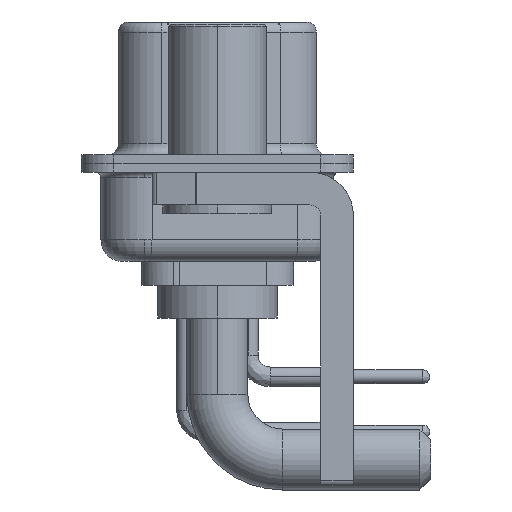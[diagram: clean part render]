
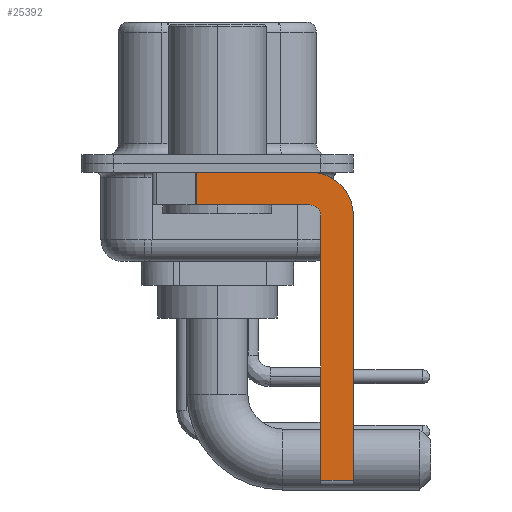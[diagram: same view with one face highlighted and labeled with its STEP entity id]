
A CAD part, left-side view. The second image highlights one B-rep face of the part: STEP entity #25392.
In plain terms, the highlighted planar face has unit normal (-1, 0, 0).
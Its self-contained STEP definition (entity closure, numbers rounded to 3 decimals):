
#277 = AXIS2_PLACEMENT_3D ( 'NONE', #25012, #14095, #2084 ) ;
#881 = VERTEX_POINT ( 'NONE', #25821 ) ;
#1530 = DIRECTION ( 'NONE',  ( 0., 0., -1. ) ) ;
#1732 = CARTESIAN_POINT ( 'NONE',  ( -2.9, -6.25, -2.4 ) ) ;
#1864 = DIRECTION ( 'NONE',  ( 0., -1., 0. ) ) ;
#2084 = DIRECTION ( 'NONE',  ( 0., 0., 1. ) ) ;
#2325 = VERTEX_POINT ( 'NONE', #13646 ) ;
#2996 = VECTOR ( 'NONE', #1864, 1000. ) ;
#3600 = ORIENTED_EDGE ( 'NONE', *, *, #15627, .F. ) ;
#5427 = DIRECTION ( 'NONE',  ( 0., 0., -1. ) ) ;
#5645 = VECTOR ( 'NONE', #12562, 1000. ) ;
#6056 = CARTESIAN_POINT ( 'NONE',  ( -2.9, -6.25, -14.55 ) ) ;
#6804 = CIRCLE ( 'NONE', #277, 0.5 ) ;
#6904 = EDGE_CURVE ( 'NONE', #26498, #11648, #24793, .T. ) ;
#7763 = ORIENTED_EDGE ( 'NONE', *, *, #18402, .F. ) ;
#7865 = CARTESIAN_POINT ( 'NONE',  ( -2.9, 3., -0.4 ) ) ;
#7997 = LINE ( 'NONE', #7865, #25179 ) ;
#8092 = VERTEX_POINT ( 'NONE', #1732 ) ;
#8400 = EDGE_LOOP ( 'NONE', ( #18350, #20462, #3600, #20736, #19593, #17802, #7763, #24963 ) ) ;
#9025 = CIRCLE ( 'NONE', #20380, 2. ) ;
#9372 = DIRECTION ( 'NONE',  ( 1., 0., 0. ) ) ;
#9666 = VERTEX_POINT ( 'NONE', #16493 ) ;
#10120 = CARTESIAN_POINT ( 'NONE',  ( -2.9, -4.25, -1.9 ) ) ;
#10349 = CARTESIAN_POINT ( 'NONE',  ( -2.9, 0.978, -1.9 ) ) ;
#11109 = DIRECTION ( 'NONE',  ( 0., 0., -1. ) ) ;
#11648 = VERTEX_POINT ( 'NONE', #6056 ) ;
#12027 = AXIS2_PLACEMENT_3D ( 'NONE', #26313, #9372, #5427 ) ;
#12562 = DIRECTION ( 'NONE',  ( 0., 1., 0. ) ) ;
#12820 = CARTESIAN_POINT ( 'NONE',  ( -2.9, -4.25, -2.4 ) ) ;
#13646 = CARTESIAN_POINT ( 'NONE',  ( -2.9, -4.25, -0.4 ) ) ;
#13947 = LINE ( 'NONE', #22413, #15837 ) ;
#14095 = DIRECTION ( 'NONE',  ( -1., 0., 0. ) ) ;
#14856 = CARTESIAN_POINT ( 'NONE',  ( -2.9, -4.75, -14.55 ) ) ;
#15075 = DIRECTION ( 'NONE',  ( 0., 0., 1. ) ) ;
#15415 = EDGE_CURVE ( 'NONE', #26498, #881, #25723, .T. ) ;
#15627 = EDGE_CURVE ( 'NONE', #25010, #16134, #26785, .T. ) ;
#15837 = VECTOR ( 'NONE', #1530, 1000. ) ;
#16134 = VERTEX_POINT ( 'NONE', #10349 ) ;
#16237 = VECTOR ( 'NONE', #11109, 1000. ) ;
#16348 = DIRECTION ( 'NONE',  ( 0., -1., 0. ) ) ;
#16493 = CARTESIAN_POINT ( 'NONE',  ( -2.9, 0.978, -0.4 ) ) ;
#17627 = CARTESIAN_POINT ( 'NONE',  ( -2.9, -4.25, -1.9 ) ) ;
#17802 = ORIENTED_EDGE ( 'NONE', *, *, #6904, .T. ) ;
#18350 = ORIENTED_EDGE ( 'NONE', *, *, #26889, .F. ) ;
#18402 = EDGE_CURVE ( 'NONE', #8092, #11648, #21763, .T. ) ;
#19593 = ORIENTED_EDGE ( 'NONE', *, *, #15415, .F. ) ;
#19669 = DIRECTION ( 'NONE',  ( 0., 0., -1. ) ) ;
#20380 = AXIS2_PLACEMENT_3D ( 'NONE', #12820, #23762, #19669 ) ;
#20462 = ORIENTED_EDGE ( 'NONE', *, *, #20621, .T. ) ;
#20585 = CARTESIAN_POINT ( 'NONE',  ( -2.9, -4.25, -14.55 ) ) ;
#20621 = EDGE_CURVE ( 'NONE', #9666, #16134, #13947, .T. ) ;
#20736 = ORIENTED_EDGE ( 'NONE', *, *, #23852, .F. ) ;
#21504 = CARTESIAN_POINT ( 'NONE',  ( -2.9, -6.25, -2.4 ) ) ;
#21633 = CARTESIAN_POINT ( 'NONE',  ( -2.9, -4.75, -14.8 ) ) ;
#21686 = PLANE ( 'NONE',  #12027 ) ;
#21763 = LINE ( 'NONE', #21504, #16237 ) ;
#22413 = CARTESIAN_POINT ( 'NONE',  ( -2.9, 0.978, -1.9 ) ) ;
#22642 = VECTOR ( 'NONE', #15075, 1000. ) ;
#23762 = DIRECTION ( 'NONE',  ( 1., 0., 0. ) ) ;
#23852 = EDGE_CURVE ( 'NONE', #881, #25010, #6804, .T. ) ;
#24793 = LINE ( 'NONE', #20585, #2996 ) ;
#24963 = ORIENTED_EDGE ( 'NONE', *, *, #26171, .F. ) ;
#25010 = VERTEX_POINT ( 'NONE', #17627 ) ;
#25012 = CARTESIAN_POINT ( 'NONE',  ( -2.9, -4.25, -2.4 ) ) ;
#25179 = VECTOR ( 'NONE', #16348, 1000. ) ;
#25392 = ADVANCED_FACE ( 'NONE', ( #26177 ), #21686, .F. ) ;
#25723 = LINE ( 'NONE', #21633, #22642 ) ;
#25821 = CARTESIAN_POINT ( 'NONE',  ( -2.9, -4.75, -2.4 ) ) ;
#26171 = EDGE_CURVE ( 'NONE', #2325, #8092, #9025, .T. ) ;
#26177 = FACE_OUTER_BOUND ( 'NONE', #8400, .T. ) ;
#26313 = CARTESIAN_POINT ( 'NONE',  ( -2.9, -4.25, -2.4 ) ) ;
#26498 = VERTEX_POINT ( 'NONE', #14856 ) ;
#26785 = LINE ( 'NONE', #10120, #5645 ) ;
#26889 = EDGE_CURVE ( 'NONE', #9666, #2325, #7997, .T. ) ;
